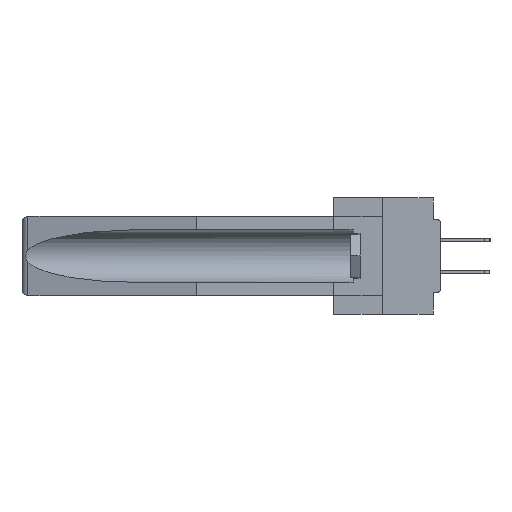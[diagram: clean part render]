
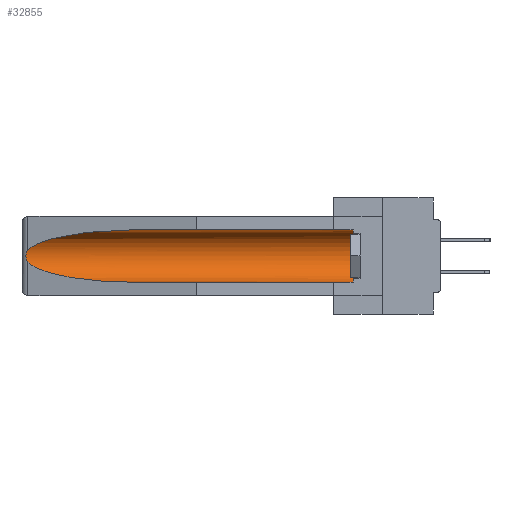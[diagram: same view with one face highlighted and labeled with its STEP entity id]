
A CAD part, left-side view. The second image highlights one B-rep face of the part: STEP entity #32855.
In plain terms, the highlighted cylindrical face has radius 2.857 mm (diameter 5.715 mm), a partial arc.
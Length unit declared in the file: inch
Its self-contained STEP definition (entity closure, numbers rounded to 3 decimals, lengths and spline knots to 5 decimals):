
#862 = CARTESIAN_POINT ( 'NONE',  ( 0.2673, 1.53269, -0.17917 ) ) ;
#1128 = EDGE_CURVE ( 'NONE', #22468, #18016, #8114, .T. ) ;
#1593 = CARTESIAN_POINT ( 'NONE',  ( 0.155, 0.126, -0.284 ) ) ;
#2272 = CARTESIAN_POINT ( 'NONE',  ( 0.155, 1.07973, -0.284 ) ) ;
#2292 = B_SPLINE_CURVE_WITH_KNOTS ( 'NONE', 3,
 ( #28056, #8727, #25284, #30821, #14444, #17175, #862, #6359, #25395, #9086 ),
 .UNSPECIFIED., .F., .F.,
 ( 4, 2, 2, 2, 4 ),
 ( 0., 0.00029, 0.00058, 0.00087, 0.00117 ),
 .UNSPECIFIED. ) ;
#2824 = CARTESIAN_POINT ( 'NONE',  ( 0.25451, 1.48313, -0.24835 ) ) ;
#3472 = LINE ( 'NONE', #28133, #35016 ) ;
#3516 = CARTESIAN_POINT ( 'NONE',  ( 0.25451, 1.48313, -0.09465 ) ) ;
#3814 =( BOUNDED_CURVE ( )  B_SPLINE_CURVE ( 3, ( #25417, #14701, #3516, #27960 ),
 .UNSPECIFIED., .F., .F. ) 
 B_SPLINE_CURVE_WITH_KNOTS ( ( 4, 4 ),
 ( 4.71239, 6.08839 ),
 .UNSPECIFIED. ) 
 CURVE ( )  GEOMETRIC_REPRESENTATION_ITEM ( )  RATIONAL_B_SPLINE_CURVE ( ( 1., 0.848, 0.848, 1. ) ) 
 REPRESENTATION_ITEM ( '' )  );
#4271 = DIRECTION ( 'NONE',  ( 0., 0., 1. ) ) ;
#6245 = CARTESIAN_POINT ( 'NONE',  ( 0.155, 1.07973, -0.059 ) ) ;
#6359 = CARTESIAN_POINT ( 'NONE',  ( 0.26655, 1.53094, -0.18657 ) ) ;
#7682 = ORIENTED_EDGE ( 'NONE', *, *, #32749, .T. ) ;
#8114 = CIRCLE ( 'NONE', #27491, 0.1125 ) ;
#8727 = CARTESIAN_POINT ( 'NONE',  ( 0.26597, 1.52961, -0.15275 ) ) ;
#8957 = EDGE_CURVE ( 'NONE', #22781, #14550, #3814, .T. ) ;
#9015 = CYLINDRICAL_SURFACE ( 'NONE', #24563, 0.1125 ) ;
#9086 = CARTESIAN_POINT ( 'NONE',  ( 0.26537, 1.52718, -0.19328 ) ) ;
#9192 = CARTESIAN_POINT ( 'NONE',  ( 0.155, -0.30754, -0.1715 ) ) ;
#9877 = CARTESIAN_POINT ( 'NONE',  ( 0.155, -0.30754, -0.059 ) ) ;
#10519 = ORIENTED_EDGE ( 'NONE', *, *, #11707, .F. ) ;
#10667 = CARTESIAN_POINT ( 'NONE',  ( 0.155, 1.07973, -0.284 ) ) ;
#10775 =( BOUNDED_CURVE ( )  B_SPLINE_CURVE ( 3, ( #16264, #2824, #24380, #10667 ),
 .UNSPECIFIED., .F., .F. ) 
 B_SPLINE_CURVE_WITH_KNOTS ( ( 4, 4 ),
 ( 0.1948, 1.5708 ),
 .UNSPECIFIED. ) 
 CURVE ( )  GEOMETRIC_REPRESENTATION_ITEM ( )  RATIONAL_B_SPLINE_CURVE ( ( 1., 0.848, 0.848, 1. ) ) 
 REPRESENTATION_ITEM ( '' )  );
#11707 = EDGE_CURVE ( 'NONE', #22468, #18410, #3472, .T. ) ;
#13158 = CARTESIAN_POINT ( 'NONE',  ( 0.155, 0.126, -0.059 ) ) ;
#13298 = DIRECTION ( 'NONE',  ( 0., 1., 0. ) ) ;
#14444 = CARTESIAN_POINT ( 'NONE',  ( 0.2675, 1.53308, -0.16763 ) ) ;
#14550 = VERTEX_POINT ( 'NONE', #23968 ) ;
#14674 = DIRECTION ( 'NONE',  ( 0., 1., 0. ) ) ;
#14701 = CARTESIAN_POINT ( 'NONE',  ( 0.21114, 1.30732, -0.059 ) ) ;
#15017 = DIRECTION ( 'NONE',  ( 0., 0., 1. ) ) ;
#15223 = DIRECTION ( 'NONE',  ( 0., 1., 0. ) ) ;
#15824 = ORIENTED_EDGE ( 'NONE', *, *, #16297, .T. ) ;
#16264 = CARTESIAN_POINT ( 'NONE',  ( 0.26537, 1.52718, -0.19328 ) ) ;
#16297 = EDGE_CURVE ( 'NONE', #17251, #18410, #10775, .T. ) ;
#17175 = CARTESIAN_POINT ( 'NONE',  ( 0.2675, 1.53308, -0.17534 ) ) ;
#17251 = VERTEX_POINT ( 'NONE', #27579 ) ;
#18016 = VERTEX_POINT ( 'NONE', #13158 ) ;
#18410 = VERTEX_POINT ( 'NONE', #2272 ) ;
#20502 = ORIENTED_EDGE ( 'NONE', *, *, #30970, .T. ) ;
#22468 = VERTEX_POINT ( 'NONE', #1593 ) ;
#22781 = VERTEX_POINT ( 'NONE', #6245 ) ;
#23293 = CARTESIAN_POINT ( 'NONE',  ( 0.155, 0.126, -0.1715 ) ) ;
#23968 = CARTESIAN_POINT ( 'NONE',  ( 0.26537, 1.52718, -0.14972 ) ) ;
#24380 = CARTESIAN_POINT ( 'NONE',  ( 0.21114, 1.30732, -0.284 ) ) ;
#24563 = AXIS2_PLACEMENT_3D ( 'NONE', #9192, #14674, #15017 ) ;
#25284 = CARTESIAN_POINT ( 'NONE',  ( 0.26654, 1.53092, -0.15636 ) ) ;
#25395 = CARTESIAN_POINT ( 'NONE',  ( 0.26597, 1.5296, -0.19026 ) ) ;
#25417 = CARTESIAN_POINT ( 'NONE',  ( 0.155, 1.07973, -0.059 ) ) ;
#25606 = FACE_OUTER_BOUND ( 'NONE', #33239, .T. ) ;
#27491 = AXIS2_PLACEMENT_3D ( 'NONE', #23293, #34514, #4271 ) ;
#27579 = CARTESIAN_POINT ( 'NONE',  ( 0.26537, 1.52718, -0.19328 ) ) ;
#27960 = CARTESIAN_POINT ( 'NONE',  ( 0.26537, 1.52718, -0.14972 ) ) ;
#28056 = CARTESIAN_POINT ( 'NONE',  ( 0.26537, 1.52718, -0.14972 ) ) ;
#28133 = CARTESIAN_POINT ( 'NONE',  ( 0.155, -0.30754, -0.284 ) ) ;
#29710 = VECTOR ( 'NONE', #15223, 39.37008 ) ;
#30544 = ORIENTED_EDGE ( 'NONE', *, *, #8957, .T. ) ;
#30565 = LINE ( 'NONE', #9877, #29710 ) ;
#30821 = CARTESIAN_POINT ( 'NONE',  ( 0.2673, 1.5327, -0.16383 ) ) ;
#30970 = EDGE_CURVE ( 'NONE', #18016, #22781, #30565, .T. ) ;
#32749 = EDGE_CURVE ( 'NONE', #14550, #17251, #2292, .T. ) ;
#32855 = ADVANCED_FACE ( 'NONE', ( #25606 ), #9015, .F. ) ;
#33239 = EDGE_LOOP ( 'NONE', ( #30544, #7682, #15824, #10519, #33733, #20502 ) ) ;
#33733 = ORIENTED_EDGE ( 'NONE', *, *, #1128, .T. ) ;
#34514 = DIRECTION ( 'NONE',  ( 0., -1., 0. ) ) ;
#35016 = VECTOR ( 'NONE', #13298, 39.37008 ) ;
